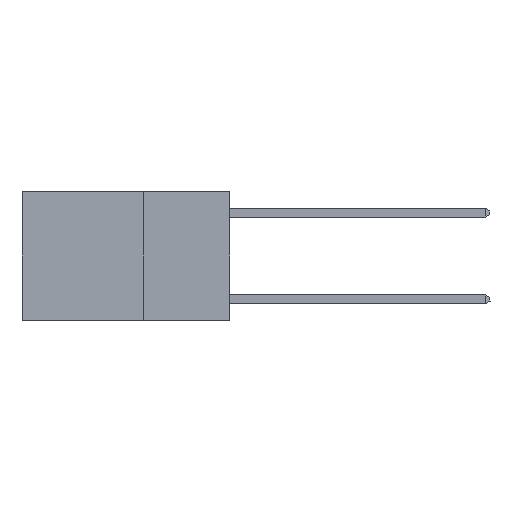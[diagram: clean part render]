
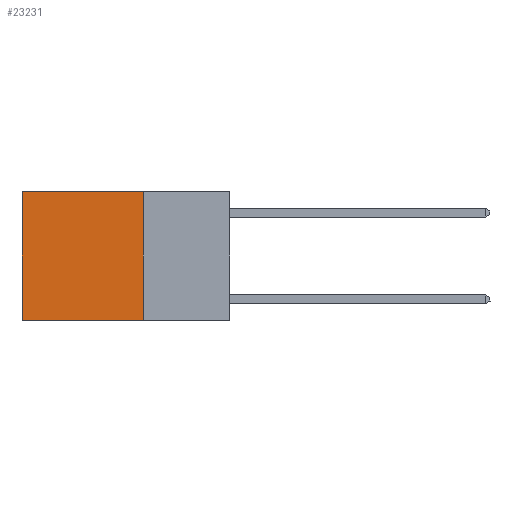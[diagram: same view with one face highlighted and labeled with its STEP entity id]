
A CAD part, left-side view. The second image highlights one B-rep face of the part: STEP entity #23231.
In plain terms, the highlighted planar face has unit normal (-1, 0, 0).
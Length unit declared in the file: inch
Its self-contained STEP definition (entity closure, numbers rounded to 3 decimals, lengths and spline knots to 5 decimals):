
#727 = DIRECTION ( 'NONE',  ( 0., 1., 0. ) ) ;
#1542 = VECTOR ( 'NONE', #12184, 39.37008 ) ;
#2413 = CARTESIAN_POINT ( 'NONE',  ( 0.2625, 0.25, 0. ) ) ;
#2575 = VECTOR ( 'NONE', #727, 39.37008 ) ;
#2804 = CARTESIAN_POINT ( 'NONE',  ( 0.2625, 0.25, -0.37 ) ) ;
#3026 = CARTESIAN_POINT ( 'NONE',  ( 0.2625, 0.25, -0.37 ) ) ;
#3775 = VECTOR ( 'NONE', #13558, 39.37008 ) ;
#4480 = VERTEX_POINT ( 'NONE', #27415 ) ;
#5100 = CARTESIAN_POINT ( 'NONE',  ( 0.2625, 0.6, -0.37 ) ) ;
#5108 = VERTEX_POINT ( 'NONE', #14116 ) ;
#7134 = FACE_OUTER_BOUND ( 'NONE', #10392, .T. ) ;
#7652 = PLANE ( 'NONE',  #15546 ) ;
#7752 = DIRECTION ( 'NONE',  ( 1., 0., 0. ) ) ;
#8025 = CARTESIAN_POINT ( 'NONE',  ( 0.2625, 0.25, 0. ) ) ;
#9522 = LINE ( 'NONE', #2413, #25714 ) ;
#10058 = LINE ( 'NONE', #8025, #1542 ) ;
#10392 = EDGE_LOOP ( 'NONE', ( #23975, #17366, #16573, #19708 ) ) ;
#10420 = EDGE_CURVE ( 'NONE', #4480, #5108, #9522, .T. ) ;
#11332 = VERTEX_POINT ( 'NONE', #5100 ) ;
#12184 = DIRECTION ( 'NONE',  ( 0., 0., -1. ) ) ;
#12355 = LINE ( 'NONE', #26436, #3775 ) ;
#13558 = DIRECTION ( 'NONE',  ( 0., 0., -1. ) ) ;
#14116 = CARTESIAN_POINT ( 'NONE',  ( 0.2625, 0.6, 0. ) ) ;
#15546 = AXIS2_PLACEMENT_3D ( 'NONE', #23031, #7752, #16717 ) ;
#16573 = ORIENTED_EDGE ( 'NONE', *, *, #19238, .F. ) ;
#16689 = VERTEX_POINT ( 'NONE', #2804 ) ;
#16717 = DIRECTION ( 'NONE',  ( 0., 0., -1. ) ) ;
#17366 = ORIENTED_EDGE ( 'NONE', *, *, #18186, .F. ) ;
#17801 = DIRECTION ( 'NONE',  ( 0., 1., 0. ) ) ;
#18186 = EDGE_CURVE ( 'NONE', #16689, #11332, #20538, .T. ) ;
#19238 = EDGE_CURVE ( 'NONE', #4480, #16689, #10058, .T. ) ;
#19708 = ORIENTED_EDGE ( 'NONE', *, *, #10420, .T. ) ;
#20538 = LINE ( 'NONE', #3026, #2575 ) ;
#23018 = EDGE_CURVE ( 'NONE', #5108, #11332, #12355, .T. ) ;
#23031 = CARTESIAN_POINT ( 'NONE',  ( 0.2625, 0.25, 0. ) ) ;
#23231 = ADVANCED_FACE ( 'NONE', ( #7134 ), #7652, .F. ) ;
#23975 = ORIENTED_EDGE ( 'NONE', *, *, #23018, .T. ) ;
#25714 = VECTOR ( 'NONE', #17801, 39.37008 ) ;
#26436 = CARTESIAN_POINT ( 'NONE',  ( 0.2625, 0.6, 0. ) ) ;
#27415 = CARTESIAN_POINT ( 'NONE',  ( 0.2625, 0.25, 0. ) ) ;
